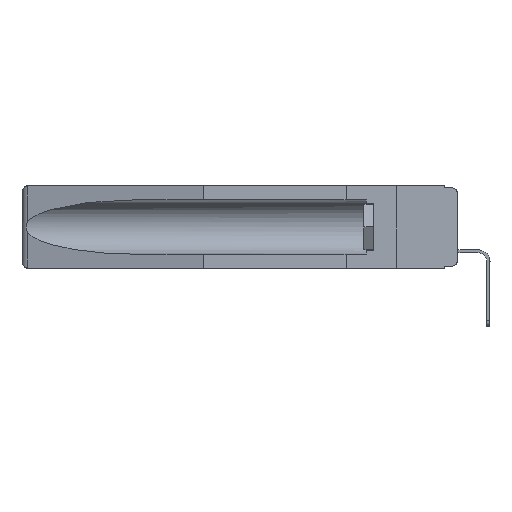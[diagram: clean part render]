
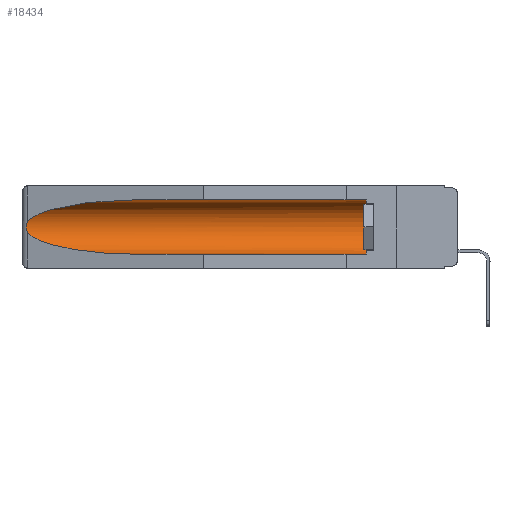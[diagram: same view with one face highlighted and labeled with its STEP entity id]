
A CAD part, left-side view. The second image highlights one B-rep face of the part: STEP entity #18434.
In plain terms, the highlighted cylindrical face has radius 2.857 mm (diameter 5.715 mm), a partial arc.
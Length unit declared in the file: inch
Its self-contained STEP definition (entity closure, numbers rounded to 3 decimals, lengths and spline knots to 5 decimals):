
#562 = VERTEX_POINT ( 'NONE', #17191 ) ;
#1184 = ORIENTED_EDGE ( 'NONE', *, *, #21652, .T. ) ;
#1299 = CARTESIAN_POINT ( 'NONE',  ( 0.26654, 1.53092, -0.15636 ) ) ;
#1457 = AXIS2_PLACEMENT_3D ( 'NONE', #12377, #1680, #7010 ) ;
#1680 = DIRECTION ( 'NONE',  ( 0., 1., 0. ) ) ;
#2106 = CARTESIAN_POINT ( 'NONE',  ( 0.155, 0.126, -0.1715 ) ) ;
#2176 = DIRECTION ( 'NONE',  ( 0., -1., 0. ) ) ;
#2891 = LINE ( 'NONE', #3915, #15426 ) ;
#3116 = CARTESIAN_POINT ( 'NONE',  ( 0.26597, 1.5296, -0.19026 ) ) ;
#3455 = CARTESIAN_POINT ( 'NONE',  ( 0.26537, 1.52718, -0.14972 ) ) ;
#3466 = VERTEX_POINT ( 'NONE', #8146 ) ;
#3514 = CARTESIAN_POINT ( 'NONE',  ( 0.26597, 1.52961, -0.15275 ) ) ;
#3597 = CARTESIAN_POINT ( 'NONE',  ( 0.2673, 1.5327, -0.16383 ) ) ;
#3754 = CARTESIAN_POINT ( 'NONE',  ( 0.26537, 1.52718, -0.19328 ) ) ;
#3915 = CARTESIAN_POINT ( 'NONE',  ( 0.155, -0.30754, -0.284 ) ) ;
#4102 =( BOUNDED_CURVE ( )  B_SPLINE_CURVE ( 3, ( #13006, #9537, #11302, #14888 ),
 .UNSPECIFIED., .F., .F. ) 
 B_SPLINE_CURVE_WITH_KNOTS ( ( 4, 4 ),
 ( 0.1948, 1.5708 ),
 .UNSPECIFIED. ) 
 CURVE ( )  GEOMETRIC_REPRESENTATION_ITEM ( )  RATIONAL_B_SPLINE_CURVE ( ( 1., 0.848, 0.848, 1. ) ) 
 REPRESENTATION_ITEM ( '' )  );
#4700 = EDGE_CURVE ( 'NONE', #7699, #6363, #2891, .T. ) ;
#4771 = CARTESIAN_POINT ( 'NONE',  ( 0.155, 1.07973, -0.059 ) ) ;
#5789 = B_SPLINE_CURVE_WITH_KNOTS ( 'NONE', 3,
 ( #16202, #3514, #1299, #3597, #16132, #17988, #7099, #14151, #3116, #3754 ),
 .UNSPECIFIED., .F., .F.,
 ( 4, 2, 2, 2, 4 ),
 ( 0., 0.00029, 0.00058, 0.00087, 0.00117 ),
 .UNSPECIFIED. ) ;
#5816 =( BOUNDED_CURVE ( )  B_SPLINE_CURVE ( 3, ( #4771, #13643, #22954, #3455 ),
 .UNSPECIFIED., .F., .F. ) 
 B_SPLINE_CURVE_WITH_KNOTS ( ( 4, 4 ),
 ( 4.71239, 6.08839 ),
 .UNSPECIFIED. ) 
 CURVE ( )  GEOMETRIC_REPRESENTATION_ITEM ( )  RATIONAL_B_SPLINE_CURVE ( ( 1., 0.848, 0.848, 1. ) ) 
 REPRESENTATION_ITEM ( '' )  );
#5983 = CARTESIAN_POINT ( 'NONE',  ( 0.155, -0.30754, -0.059 ) ) ;
#6363 = VERTEX_POINT ( 'NONE', #15904 ) ;
#6466 = ORIENTED_EDGE ( 'NONE', *, *, #10716, .T. ) ;
#6502 = EDGE_CURVE ( 'NONE', #18242, #6363, #4102, .T. ) ;
#7010 = DIRECTION ( 'NONE',  ( 0., 0., 1. ) ) ;
#7099 = CARTESIAN_POINT ( 'NONE',  ( 0.2673, 1.53269, -0.17917 ) ) ;
#7699 = VERTEX_POINT ( 'NONE', #21094 ) ;
#8146 = CARTESIAN_POINT ( 'NONE',  ( 0.155, 1.07973, -0.059 ) ) ;
#8423 = ORIENTED_EDGE ( 'NONE', *, *, #8677, .T. ) ;
#8677 = EDGE_CURVE ( 'NONE', #7699, #562, #11056, .T. ) ;
#8828 = ORIENTED_EDGE ( 'NONE', *, *, #4700, .F. ) ;
#9537 = CARTESIAN_POINT ( 'NONE',  ( 0.25451, 1.48313, -0.24835 ) ) ;
#10116 = ORIENTED_EDGE ( 'NONE', *, *, #11425, .T. ) ;
#10716 = EDGE_CURVE ( 'NONE', #14566, #18242, #5789, .T. ) ;
#11056 = CIRCLE ( 'NONE', #18773, 0.1125 ) ;
#11302 = CARTESIAN_POINT ( 'NONE',  ( 0.21114, 1.30732, -0.284 ) ) ;
#11425 = EDGE_CURVE ( 'NONE', #562, #3466, #16954, .T. ) ;
#12377 = CARTESIAN_POINT ( 'NONE',  ( 0.155, -0.30754, -0.1715 ) ) ;
#13006 = CARTESIAN_POINT ( 'NONE',  ( 0.26537, 1.52718, -0.19328 ) ) ;
#13643 = CARTESIAN_POINT ( 'NONE',  ( 0.21114, 1.30732, -0.059 ) ) ;
#14151 = CARTESIAN_POINT ( 'NONE',  ( 0.26655, 1.53094, -0.18657 ) ) ;
#14208 = EDGE_LOOP ( 'NONE', ( #1184, #6466, #22636, #8828, #8423, #10116 ) ) ;
#14560 = DIRECTION ( 'NONE',  ( 0., 0., 1. ) ) ;
#14566 = VERTEX_POINT ( 'NONE', #15168 ) ;
#14888 = CARTESIAN_POINT ( 'NONE',  ( 0.155, 1.07973, -0.284 ) ) ;
#14932 = DIRECTION ( 'NONE',  ( 0., 1., 0. ) ) ;
#15168 = CARTESIAN_POINT ( 'NONE',  ( 0.26537, 1.52718, -0.14972 ) ) ;
#15426 = VECTOR ( 'NONE', #21936, 39.37008 ) ;
#15904 = CARTESIAN_POINT ( 'NONE',  ( 0.155, 1.07973, -0.284 ) ) ;
#16132 = CARTESIAN_POINT ( 'NONE',  ( 0.2675, 1.53308, -0.16763 ) ) ;
#16202 = CARTESIAN_POINT ( 'NONE',  ( 0.26537, 1.52718, -0.14972 ) ) ;
#16954 = LINE ( 'NONE', #5983, #19750 ) ;
#17191 = CARTESIAN_POINT ( 'NONE',  ( 0.155, 0.126, -0.059 ) ) ;
#17364 = FACE_OUTER_BOUND ( 'NONE', #14208, .T. ) ;
#17879 = CYLINDRICAL_SURFACE ( 'NONE', #1457, 0.1125 ) ;
#17988 = CARTESIAN_POINT ( 'NONE',  ( 0.2675, 1.53308, -0.17534 ) ) ;
#18242 = VERTEX_POINT ( 'NONE', #19168 ) ;
#18434 = ADVANCED_FACE ( 'NONE', ( #17364 ), #17879, .F. ) ;
#18773 = AXIS2_PLACEMENT_3D ( 'NONE', #2106, #2176, #14560 ) ;
#19168 = CARTESIAN_POINT ( 'NONE',  ( 0.26537, 1.52718, -0.19328 ) ) ;
#19750 = VECTOR ( 'NONE', #14932, 39.37008 ) ;
#21094 = CARTESIAN_POINT ( 'NONE',  ( 0.155, 0.126, -0.284 ) ) ;
#21652 = EDGE_CURVE ( 'NONE', #3466, #14566, #5816, .T. ) ;
#21936 = DIRECTION ( 'NONE',  ( 0., 1., 0. ) ) ;
#22636 = ORIENTED_EDGE ( 'NONE', *, *, #6502, .T. ) ;
#22954 = CARTESIAN_POINT ( 'NONE',  ( 0.25451, 1.48313, -0.09465 ) ) ;
